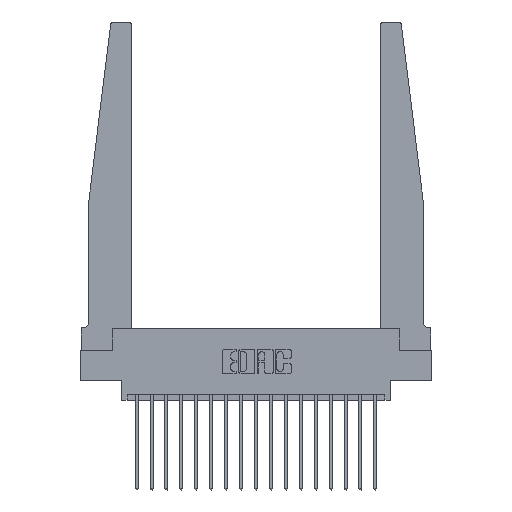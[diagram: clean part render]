
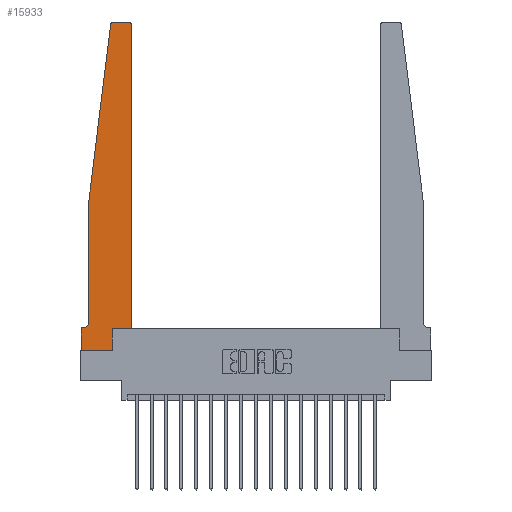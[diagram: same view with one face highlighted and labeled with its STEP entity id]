
A CAD part, top view. The second image highlights one B-rep face of the part: STEP entity #15933.
In plain terms, the highlighted planar face has unit normal (0, 0, 1).
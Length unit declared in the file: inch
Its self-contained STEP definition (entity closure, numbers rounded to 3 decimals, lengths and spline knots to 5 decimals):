
#498 = EDGE_CURVE ( 'NONE', #8527, #16595, #7457, .T. ) ;
#603 = CARTESIAN_POINT ( 'NONE',  ( 0.015, 0.1875, 0.37 ) ) ;
#879 = CARTESIAN_POINT ( 'NONE',  ( 0.425, 0.18, 0.37 ) ) ;
#915 = EDGE_CURVE ( 'NONE', #6776, #1364, #5329, .T. ) ;
#1014 = VERTEX_POINT ( 'NONE', #879 ) ;
#1209 = CARTESIAN_POINT ( 'NONE',  ( 0., 0., 0.37 ) ) ;
#1364 = VERTEX_POINT ( 'NONE', #14972 ) ;
#1569 = VERTEX_POINT ( 'NONE', #603 ) ;
#1667 = ORIENTED_EDGE ( 'NONE', *, *, #8018, .T. ) ;
#1708 = EDGE_CURVE ( 'NONE', #15744, #5942, #16292, .T. ) ;
#1732 = CARTESIAN_POINT ( 'NONE',  ( 0.425, 2.72, 0.37 ) ) ;
#2482 = ORIENTED_EDGE ( 'NONE', *, *, #7061, .T. ) ;
#2515 = CARTESIAN_POINT ( 'NONE',  ( 0., 0.1875, 0.37 ) ) ;
#2600 = DIRECTION ( 'NONE',  ( 0., 0., 1. ) ) ;
#2840 = ORIENTED_EDGE ( 'NONE', *, *, #8381, .T. ) ;
#3047 = CARTESIAN_POINT ( 'NONE',  ( 0., 0.1875, 0.37 ) ) ;
#3503 = CARTESIAN_POINT ( 'NONE',  ( 0.065, 1.25, 0.37 ) ) ;
#3831 = DIRECTION ( 'NONE',  ( 1., 0., 0. ) ) ;
#3854 = CARTESIAN_POINT ( 'NONE',  ( 0.395, 2.75, 0.37 ) ) ;
#3954 = AXIS2_PLACEMENT_3D ( 'NONE', #4996, #15425, #6490 ) ;
#3989 = CARTESIAN_POINT ( 'NONE',  ( 0.2605, 0.18, 0.37 ) ) ;
#4035 = AXIS2_PLACEMENT_3D ( 'NONE', #8878, #19357, #10372 ) ;
#4430 = CARTESIAN_POINT ( 'NONE',  ( 0.065, 1.25, 0.37 ) ) ;
#4561 = EDGE_CURVE ( 'NONE', #7852, #14451, #7795, .T. ) ;
#4996 = CARTESIAN_POINT ( 'NONE',  ( 0.015, 0.2375, 0.37 ) ) ;
#5208 = EDGE_CURVE ( 'NONE', #1014, #8527, #15428, .T. ) ;
#5329 = LINE ( 'NONE', #6448, #8818 ) ;
#5546 = PLANE ( 'NONE',  #7717 ) ;
#5758 = CARTESIAN_POINT ( 'NONE',  ( 0.2605, 0.18, 0.37 ) ) ;
#5942 = VERTEX_POINT ( 'NONE', #3989 ) ;
#6142 = LINE ( 'NONE', #1209, #9629 ) ;
#6157 = CIRCLE ( 'NONE', #4035, 0.03 ) ;
#6448 = CARTESIAN_POINT ( 'NONE',  ( 0., 0., 0.37 ) ) ;
#6455 = LINE ( 'NONE', #7404, #17901 ) ;
#6490 = DIRECTION ( 'NONE',  ( -1., 0., 0. ) ) ;
#6776 = VERTEX_POINT ( 'NONE', #3047 ) ;
#7015 = CARTESIAN_POINT ( 'NONE',  ( 0.27653, 2.75, 0.37 ) ) ;
#7042 = VECTOR ( 'NONE', #8086, 39.37008 ) ;
#7060 = DIRECTION ( 'NONE',  ( 1., 0., 0. ) ) ;
#7061 = EDGE_CURVE ( 'NONE', #16595, #8816, #13248, .T. ) ;
#7404 = CARTESIAN_POINT ( 'NONE',  ( 0.065, 0.1875, 0.37 ) ) ;
#7457 = CIRCLE ( 'NONE', #18443, 0.03 ) ;
#7471 = DIRECTION ( 'NONE',  ( -0.122, -0.992, 0. ) ) ;
#7605 = VERTEX_POINT ( 'NONE', #17334 ) ;
#7717 = AXIS2_PLACEMENT_3D ( 'NONE', #2515, #15979, #7060 ) ;
#7795 = LINE ( 'NONE', #3503, #11735 ) ;
#7852 = VERTEX_POINT ( 'NONE', #18054 ) ;
#7952 = EDGE_LOOP ( 'NONE', ( #2482, #18473, #2840, #13337, #1667, #8062, #15650, #16957, #18155, #12237, #16099, #18686 ) ) ;
#8018 = EDGE_CURVE ( 'NONE', #14451, #1569, #10445, .T. ) ;
#8062 = ORIENTED_EDGE ( 'NONE', *, *, #13118, .T. ) ;
#8086 = DIRECTION ( 'NONE',  ( 0., 1., 0. ) ) ;
#8381 = EDGE_CURVE ( 'NONE', #7605, #7852, #15807, .T. ) ;
#8527 = VERTEX_POINT ( 'NONE', #1732 ) ;
#8756 = DIRECTION ( 'NONE',  ( 0., 1., 0. ) ) ;
#8816 = VERTEX_POINT ( 'NONE', #7015 ) ;
#8818 = VECTOR ( 'NONE', #10861, 39.37008 ) ;
#8878 = CARTESIAN_POINT ( 'NONE',  ( 0.27653, 2.72, 0.37 ) ) ;
#9629 = VECTOR ( 'NONE', #19140, 39.37008 ) ;
#10289 = LINE ( 'NONE', #17303, #18240 ) ;
#10328 = DIRECTION ( 'NONE',  ( -1., 0., 0. ) ) ;
#10372 = DIRECTION ( 'NONE',  ( 1., 0., 0. ) ) ;
#10445 = CIRCLE ( 'NONE', #3954, 0.05 ) ;
#10861 = DIRECTION ( 'NONE',  ( 0., -1., 0. ) ) ;
#11735 = VECTOR ( 'NONE', #15483, 39.37008 ) ;
#11821 = VECTOR ( 'NONE', #7471, 39.37008 ) ;
#11843 = VECTOR ( 'NONE', #8756, 39.37008 ) ;
#12237 = ORIENTED_EDGE ( 'NONE', *, *, #17148, .T. ) ;
#12776 = VECTOR ( 'NONE', #17085, 39.37008 ) ;
#13118 = EDGE_CURVE ( 'NONE', #1569, #6776, #6455, .T. ) ;
#13183 = CARTESIAN_POINT ( 'NONE',  ( 0.395, 2.72, 0.37 ) ) ;
#13248 = LINE ( 'NONE', #15594, #12776 ) ;
#13337 = ORIENTED_EDGE ( 'NONE', *, *, #4561, .T. ) ;
#14451 = VERTEX_POINT ( 'NONE', #18451 ) ;
#14972 = CARTESIAN_POINT ( 'NONE',  ( 0., 0., 0.37 ) ) ;
#15425 = DIRECTION ( 'NONE',  ( 0., 0., -1. ) ) ;
#15428 = LINE ( 'NONE', #15456, #7042 ) ;
#15456 = CARTESIAN_POINT ( 'NONE',  ( 0.425, 0.18, 0.37 ) ) ;
#15482 = FACE_OUTER_BOUND ( 'NONE', #7952, .T. ) ;
#15483 = DIRECTION ( 'NONE',  ( 0., -1., 0. ) ) ;
#15491 = EDGE_CURVE ( 'NONE', #8816, #7605, #6157, .T. ) ;
#15594 = CARTESIAN_POINT ( 'NONE',  ( 0.25, 2.75, 0.37 ) ) ;
#15650 = ORIENTED_EDGE ( 'NONE', *, *, #915, .T. ) ;
#15744 = VERTEX_POINT ( 'NONE', #17088 ) ;
#15807 = LINE ( 'NONE', #4430, #11821 ) ;
#15933 = ADVANCED_FACE ( 'NONE', ( #15482 ), #5546, .T. ) ;
#15979 = DIRECTION ( 'NONE',  ( 0., 0., 1. ) ) ;
#16006 = EDGE_CURVE ( 'NONE', #1364, #15744, #6142, .T. ) ;
#16099 = ORIENTED_EDGE ( 'NONE', *, *, #5208, .T. ) ;
#16292 = LINE ( 'NONE', #5758, #11843 ) ;
#16385 = DIRECTION ( 'NONE',  ( 1., 0., 0. ) ) ;
#16595 = VERTEX_POINT ( 'NONE', #3854 ) ;
#16957 = ORIENTED_EDGE ( 'NONE', *, *, #16006, .T. ) ;
#17085 = DIRECTION ( 'NONE',  ( -1., 0., 0. ) ) ;
#17088 = CARTESIAN_POINT ( 'NONE',  ( 0.2605, 0., 0.37 ) ) ;
#17148 = EDGE_CURVE ( 'NONE', #5942, #1014, #10289, .T. ) ;
#17303 = CARTESIAN_POINT ( 'NONE',  ( 0.425, 0.18, 0.37 ) ) ;
#17334 = CARTESIAN_POINT ( 'NONE',  ( 0.24675, 2.72367, 0.37 ) ) ;
#17901 = VECTOR ( 'NONE', #10328, 39.37008 ) ;
#18054 = CARTESIAN_POINT ( 'NONE',  ( 0.065, 1.25, 0.37 ) ) ;
#18155 = ORIENTED_EDGE ( 'NONE', *, *, #1708, .T. ) ;
#18240 = VECTOR ( 'NONE', #3831, 39.37008 ) ;
#18443 = AXIS2_PLACEMENT_3D ( 'NONE', #13183, #2600, #16385 ) ;
#18451 = CARTESIAN_POINT ( 'NONE',  ( 0.065, 0.2375, 0.37 ) ) ;
#18473 = ORIENTED_EDGE ( 'NONE', *, *, #15491, .T. ) ;
#18686 = ORIENTED_EDGE ( 'NONE', *, *, #498, .T. ) ;
#19140 = DIRECTION ( 'NONE',  ( 1., 0., 0. ) ) ;
#19357 = DIRECTION ( 'NONE',  ( 0., 0., 1. ) ) ;
